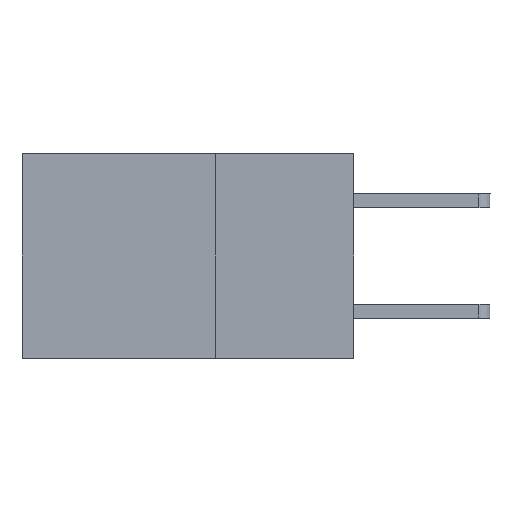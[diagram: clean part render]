
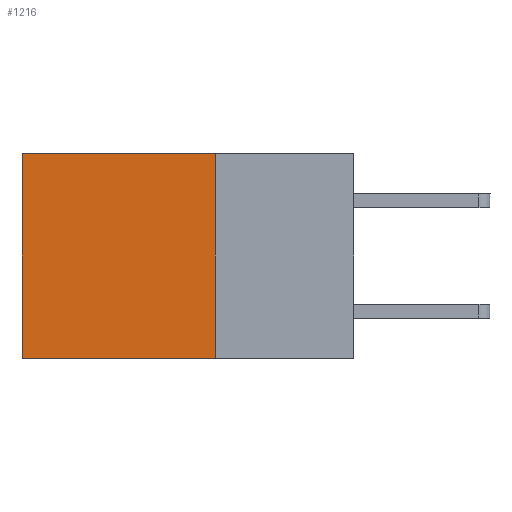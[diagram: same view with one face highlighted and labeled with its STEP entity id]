
A CAD part, left-side view. The second image highlights one B-rep face of the part: STEP entity #1216.
In plain terms, the highlighted planar face has unit normal (-1, 0, 0).
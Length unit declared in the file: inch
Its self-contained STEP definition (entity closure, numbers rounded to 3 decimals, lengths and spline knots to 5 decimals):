
#349 = VERTEX_POINT ( 'NONE', #3900 ) ;
#428 = DIRECTION ( 'NONE',  ( 1., 0., 0. ) ) ;
#589 = DIRECTION ( 'NONE',  ( 0., 0., -1. ) ) ;
#1012 = EDGE_CURVE ( 'NONE', #349, #3194, #4407, .T. ) ;
#1216 = ADVANCED_FACE ( 'NONE', ( #4079 ), #6193, .F. ) ;
#1816 = CARTESIAN_POINT ( 'NONE',  ( 0.2875, 0.25, 0. ) ) ;
#1952 = DIRECTION ( 'NONE',  ( 0., 1., 0. ) ) ;
#2060 = EDGE_LOOP ( 'NONE', ( #3928, #2562, #2791, #2719 ) ) ;
#2268 = CARTESIAN_POINT ( 'NONE',  ( 0.2875, 0.6, 0. ) ) ;
#2483 = CARTESIAN_POINT ( 'NONE',  ( 0.2875, 0.25, -0.37 ) ) ;
#2562 = ORIENTED_EDGE ( 'NONE', *, *, #1012, .F. ) ;
#2673 = DIRECTION ( 'NONE',  ( 0., 0., -1. ) ) ;
#2719 = ORIENTED_EDGE ( 'NONE', *, *, #5319, .T. ) ;
#2791 = ORIENTED_EDGE ( 'NONE', *, *, #7850, .F. ) ;
#2793 = LINE ( 'NONE', #1816, #7995 ) ;
#3055 = VECTOR ( 'NONE', #2673, 39.37008 ) ;
#3100 = VECTOR ( 'NONE', #4972, 39.37008 ) ;
#3194 = VERTEX_POINT ( 'NONE', #5600 ) ;
#3387 = CARTESIAN_POINT ( 'NONE',  ( 0.2875, 0.25, 0. ) ) ;
#3900 = CARTESIAN_POINT ( 'NONE',  ( 0.2875, 0.25, -0.37 ) ) ;
#3928 = ORIENTED_EDGE ( 'NONE', *, *, #5046, .T. ) ;
#4079 = FACE_OUTER_BOUND ( 'NONE', #2060, .T. ) ;
#4407 = LINE ( 'NONE', #2483, #7858 ) ;
#4972 = DIRECTION ( 'NONE',  ( 0., 0., -1. ) ) ;
#5046 = EDGE_CURVE ( 'NONE', #6924, #3194, #8311, .T. ) ;
#5319 = EDGE_CURVE ( 'NONE', #8106, #6924, #2793, .T. ) ;
#5484 = CARTESIAN_POINT ( 'NONE',  ( 0.2875, 0.25, 0. ) ) ;
#5600 = CARTESIAN_POINT ( 'NONE',  ( 0.2875, 0.6, -0.37 ) ) ;
#6193 = PLANE ( 'NONE',  #7452 ) ;
#6480 = DIRECTION ( 'NONE',  ( 0., 1., 0. ) ) ;
#6590 = CARTESIAN_POINT ( 'NONE',  ( 0.2875, 0.25, 0. ) ) ;
#6924 = VERTEX_POINT ( 'NONE', #8169 ) ;
#7452 = AXIS2_PLACEMENT_3D ( 'NONE', #3387, #428, #589 ) ;
#7850 = EDGE_CURVE ( 'NONE', #8106, #349, #8262, .T. ) ;
#7858 = VECTOR ( 'NONE', #1952, 39.37008 ) ;
#7995 = VECTOR ( 'NONE', #6480, 39.37008 ) ;
#8106 = VERTEX_POINT ( 'NONE', #5484 ) ;
#8169 = CARTESIAN_POINT ( 'NONE',  ( 0.2875, 0.6, 0. ) ) ;
#8262 = LINE ( 'NONE', #6590, #3055 ) ;
#8311 = LINE ( 'NONE', #2268, #3100 ) ;
